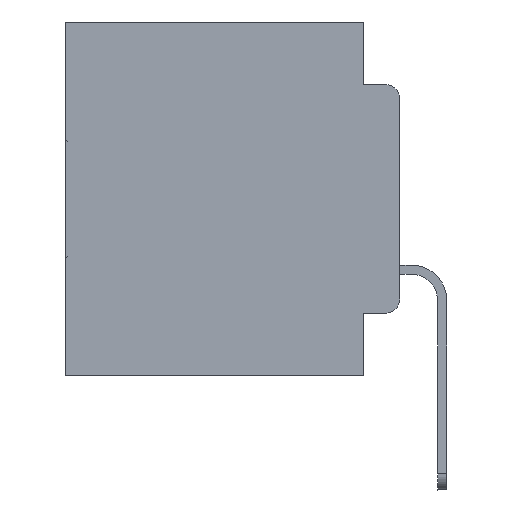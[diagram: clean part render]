
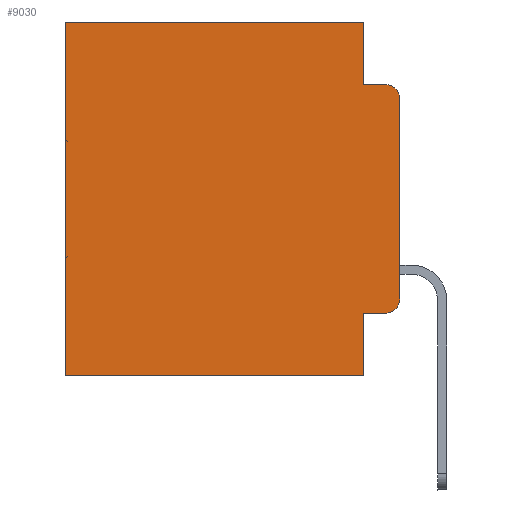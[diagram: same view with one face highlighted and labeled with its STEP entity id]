
A CAD part, left-side view. The second image highlights one B-rep face of the part: STEP entity #9030.
In plain terms, the highlighted planar face has unit normal (-1, 0, 0).
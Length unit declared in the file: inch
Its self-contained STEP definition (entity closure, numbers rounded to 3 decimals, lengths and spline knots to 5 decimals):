
#80 = ORIENTED_EDGE ( 'NONE', *, *, #25664, .F. ) ;
#903 = DIRECTION ( 'NONE',  ( 1., 0., 0. ) ) ;
#1092 = CARTESIAN_POINT ( 'NONE',  ( 0.298, 0.051, 0. ) ) ;
#1351 = CARTESIAN_POINT ( 'NONE',  ( 0.298, 0., -0.1085 ) ) ;
#2317 = ORIENTED_EDGE ( 'NONE', *, *, #2495, .F. ) ;
#2330 = VECTOR ( 'NONE', #11724, 39.37008 ) ;
#2427 = VECTOR ( 'NONE', #15680, 39.37008 ) ;
#2495 = EDGE_CURVE ( 'NONE', #4809, #25878, #29070, .T. ) ;
#3461 = LINE ( 'NONE', #29829, #24492 ) ;
#3558 = DIRECTION ( 'NONE',  ( 0., 0., -1. ) ) ;
#4055 = VERTEX_POINT ( 'NONE', #1351 ) ;
#4454 = ORIENTED_EDGE ( 'NONE', *, *, #20067, .T. ) ;
#4630 = DIRECTION ( 'NONE',  ( 0., 1., 0. ) ) ;
#4636 = VECTOR ( 'NONE', #19449, 39.37008 ) ;
#4809 = VERTEX_POINT ( 'NONE', #20946 ) ;
#5419 = ORIENTED_EDGE ( 'NONE', *, *, #10478, .T. ) ;
#5611 = DIRECTION ( 'NONE',  ( 0., 0., -1. ) ) ;
#5629 = ORIENTED_EDGE ( 'NONE', *, *, #18756, .T. ) ;
#5770 = LINE ( 'NONE', #22370, #22834 ) ;
#6509 = CARTESIAN_POINT ( 'NONE',  ( 0.298, 0.473, 0. ) ) ;
#6643 = EDGE_CURVE ( 'NONE', #16184, #4809, #24692, .T. ) ;
#6786 = CARTESIAN_POINT ( 'NONE',  ( 0.298, 0.051, 0. ) ) ;
#8216 = VECTOR ( 'NONE', #9347, 39.37008 ) ;
#8647 = DIRECTION ( 'NONE',  ( 0., 0., -1. ) ) ;
#8692 = EDGE_CURVE ( 'NONE', #25271, #27404, #5770, .T. ) ;
#9030 = ADVANCED_FACE ( 'NONE', ( #23890 ), #12102, .F. ) ;
#9203 = AXIS2_PLACEMENT_3D ( 'NONE', #20007, #15355, #3558 ) ;
#9337 = DIRECTION ( 'NONE',  ( 0., 0., -1. ) ) ;
#9347 = DIRECTION ( 'NONE',  ( 0., -1., 0. ) ) ;
#9355 = EDGE_LOOP ( 'NONE', ( #18978, #5419, #80, #26792, #5629, #4454, #2317, #15652, #9587, #29871 ) ) ;
#9587 = ORIENTED_EDGE ( 'NONE', *, *, #22394, .T. ) ;
#10463 = DIRECTION ( 'NONE',  ( 0., 0., -1. ) ) ;
#10478 = EDGE_CURVE ( 'NONE', #4055, #22316, #25051, .T. ) ;
#11571 = VECTOR ( 'NONE', #4630, 39.37008 ) ;
#11724 = DIRECTION ( 'NONE',  ( 0., -1., 0. ) ) ;
#12102 = PLANE ( 'NONE',  #12827 ) ;
#12400 = CIRCLE ( 'NONE', #30227, 0.02 ) ;
#12827 = AXIS2_PLACEMENT_3D ( 'NONE', #21560, #903, #17057 ) ;
#13174 = VERTEX_POINT ( 'NONE', #20244 ) ;
#13769 = CARTESIAN_POINT ( 'NONE',  ( 0.298, 0.02, -0.3915 ) ) ;
#15355 = DIRECTION ( 'NONE',  ( -1., 0., 0. ) ) ;
#15372 = CARTESIAN_POINT ( 'NONE',  ( 0.298, 0., -0.3915 ) ) ;
#15652 = ORIENTED_EDGE ( 'NONE', *, *, #6643, .F. ) ;
#15680 = DIRECTION ( 'NONE',  ( 0., 0., -1. ) ) ;
#16184 = VERTEX_POINT ( 'NONE', #18247 ) ;
#17057 = DIRECTION ( 'NONE',  ( 0., 0., -1. ) ) ;
#18247 = CARTESIAN_POINT ( 'NONE',  ( 0.298, 0.051, -0.4115 ) ) ;
#18489 = CARTESIAN_POINT ( 'NONE',  ( 0.298, 0.051, -0.4115 ) ) ;
#18756 = EDGE_CURVE ( 'NONE', #25271, #27622, #25124, .T. ) ;
#18939 = LINE ( 'NONE', #28404, #22962 ) ;
#18978 = ORIENTED_EDGE ( 'NONE', *, *, #21039, .F. ) ;
#19449 = DIRECTION ( 'NONE',  ( 0., 1., 0. ) ) ;
#19918 = CARTESIAN_POINT ( 'NONE',  ( 0.298, 0.02, -0.0885 ) ) ;
#20007 = CARTESIAN_POINT ( 'NONE',  ( 0.298, 0.02, -0.1085 ) ) ;
#20067 = EDGE_CURVE ( 'NONE', #27622, #25878, #18939, .T. ) ;
#20244 = CARTESIAN_POINT ( 'NONE',  ( 0.298, 0.02, -0.4115 ) ) ;
#20946 = CARTESIAN_POINT ( 'NONE',  ( 0.298, 0.051, -0.5 ) ) ;
#21039 = EDGE_CURVE ( 'NONE', #4055, #28668, #3461, .T. ) ;
#21278 = LINE ( 'NONE', #18489, #8216 ) ;
#21560 = CARTESIAN_POINT ( 'NONE',  ( 0.298, 0., 0. ) ) ;
#22316 = VERTEX_POINT ( 'NONE', #19918 ) ;
#22370 = CARTESIAN_POINT ( 'NONE',  ( 0.298, 0.051, 0. ) ) ;
#22394 = EDGE_CURVE ( 'NONE', #16184, #13174, #21278, .T. ) ;
#22834 = VECTOR ( 'NONE', #5611, 39.37008 ) ;
#22962 = VECTOR ( 'NONE', #9337, 39.37008 ) ;
#23206 = CARTESIAN_POINT ( 'NONE',  ( 0.298, 0.051, -0.0885 ) ) ;
#23890 = FACE_OUTER_BOUND ( 'NONE', #9355, .T. ) ;
#24115 = CARTESIAN_POINT ( 'NONE',  ( 0.298, 0.473, -0.5 ) ) ;
#24492 = VECTOR ( 'NONE', #10463, 39.37008 ) ;
#24692 = LINE ( 'NONE', #1092, #2427 ) ;
#25051 = CIRCLE ( 'NONE', #9203, 0.02 ) ;
#25124 = LINE ( 'NONE', #28519, #11571 ) ;
#25271 = VERTEX_POINT ( 'NONE', #6786 ) ;
#25664 = EDGE_CURVE ( 'NONE', #27404, #22316, #27862, .T. ) ;
#25878 = VERTEX_POINT ( 'NONE', #24115 ) ;
#26132 = CARTESIAN_POINT ( 'NONE',  ( 0.298, 0., -0.5 ) ) ;
#26792 = ORIENTED_EDGE ( 'NONE', *, *, #8692, .F. ) ;
#27404 = VERTEX_POINT ( 'NONE', #28714 ) ;
#27622 = VERTEX_POINT ( 'NONE', #6509 ) ;
#27736 = DIRECTION ( 'NONE',  ( -1., 0., 0. ) ) ;
#27862 = LINE ( 'NONE', #23206, #2330 ) ;
#28404 = CARTESIAN_POINT ( 'NONE',  ( 0.298, 0.473, 0. ) ) ;
#28519 = CARTESIAN_POINT ( 'NONE',  ( 0.298, 0., 0. ) ) ;
#28668 = VERTEX_POINT ( 'NONE', #15372 ) ;
#28714 = CARTESIAN_POINT ( 'NONE',  ( 0.298, 0.051, -0.0885 ) ) ;
#29070 = LINE ( 'NONE', #26132, #4636 ) ;
#29393 = EDGE_CURVE ( 'NONE', #13174, #28668, #12400, .T. ) ;
#29829 = CARTESIAN_POINT ( 'NONE',  ( 0.298, 0., 0. ) ) ;
#29871 = ORIENTED_EDGE ( 'NONE', *, *, #29393, .T. ) ;
#30227 = AXIS2_PLACEMENT_3D ( 'NONE', #13769, #27736, #8647 ) ;
